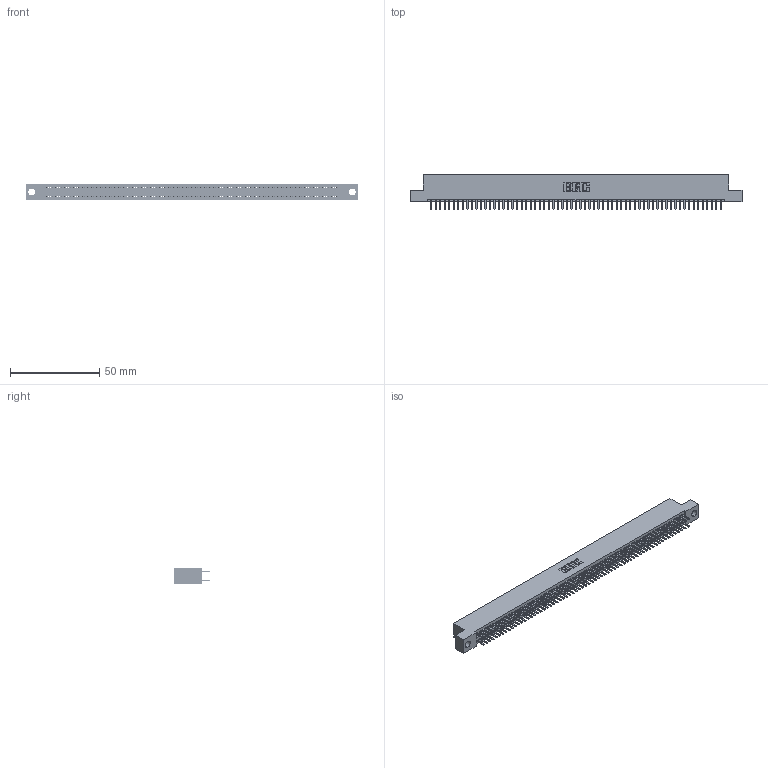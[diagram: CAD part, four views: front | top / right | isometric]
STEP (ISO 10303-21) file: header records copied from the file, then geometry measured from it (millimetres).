
FILE_DESCRIPTION (( 'STEP AP203' ), '1' );
FILE_NAME ('395-130-520-204.STEP', '2021-06-18T00:03:09', ( '' ), ( '' ), 'SwSTEP 2.0', 'SolidWorks 2020', '' );
FILE_SCHEMA (( 'CONFIG_CONTROL_DESIGN' ));
Length unit declared in the file: inch
Products named in the file (3): 345 Part_Flush Mounting Lugs - 0.156 Dia-TI; 395-130-520-204; 345-292-001_345-293-120
Assembly tree (131 placements, depth 2):
  395-130-520-204
    345 Part_Flush Mounting Lugs - 0.156 Dia-TI
    345-292-001_345-293-120  x130
Bounding box: 186.31 x 19.68 x 9.4 mm (x, y, z)
Volume: 18148.6 mm3; surface area: 27002.2 mm2
Topology: 131 solids, 131 shells, 7160 faces, 20787 edges, 13510 vertices
Faces by surface type: plane 4644, cylinder 2516
Entity records: 48437 total; most frequent: CARTESIAN_POINT 8114, ORIENTED_EDGE 8034, DIRECTION 7113, EDGE_CURVE 4017, VECTOR 3621, LINE 3621, VERTEX_POINT 2674, AXIS2_PLACEMENT_3D 1746
